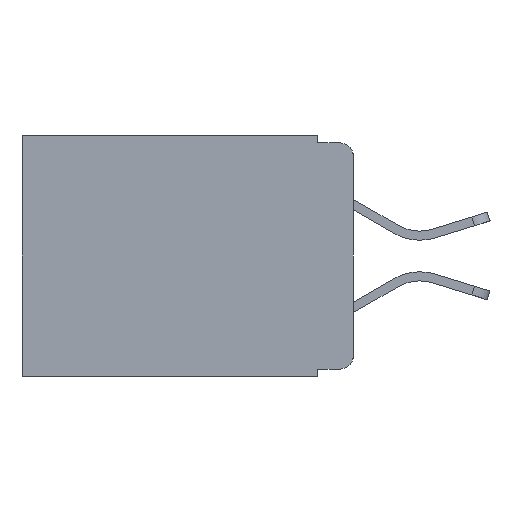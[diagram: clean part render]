
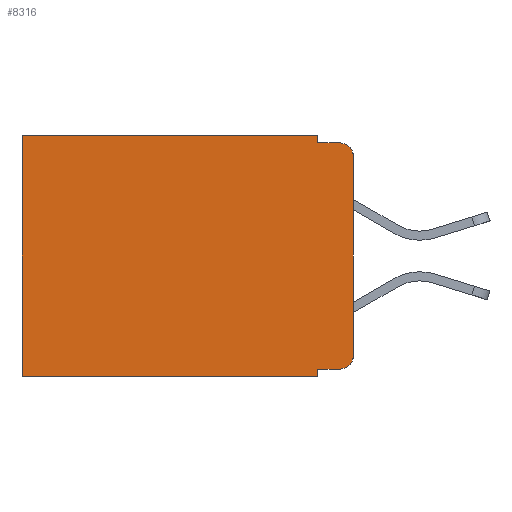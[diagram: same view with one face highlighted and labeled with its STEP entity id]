
A CAD part, left-side view. The second image highlights one B-rep face of the part: STEP entity #8316.
In plain terms, the highlighted planar face has unit normal (-1, 0, 0).
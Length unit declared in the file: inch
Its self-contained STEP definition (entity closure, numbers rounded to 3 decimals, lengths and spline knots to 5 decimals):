
#5 = CARTESIAN_POINT ( 'NONE',  ( 0.298, 0.051, 0. ) ) ;
#56 = ORIENTED_EDGE ( 'NONE', *, *, #6214, .F. ) ;
#148 = CARTESIAN_POINT ( 'NONE',  ( 0.298, 0.051, -0.343 ) ) ;
#188 = ORIENTED_EDGE ( 'NONE', *, *, #1079, .T. ) ;
#370 = VERTEX_POINT ( 'NONE', #11473 ) ;
#743 = CARTESIAN_POINT ( 'NONE',  ( 0.298, 0.02, -0.01 ) ) ;
#910 = ORIENTED_EDGE ( 'NONE', *, *, #11349, .F. ) ;
#989 = CARTESIAN_POINT ( 'NONE',  ( 0.298, 0.473, 0. ) ) ;
#1079 = EDGE_CURVE ( 'NONE', #370, #7854, #6507, .T. ) ;
#1221 = CARTESIAN_POINT ( 'NONE',  ( 0.298, 0., -0.343 ) ) ;
#1286 = VECTOR ( 'NONE', #9434, 39.37008 ) ;
#1333 = VERTEX_POINT ( 'NONE', #9067 ) ;
#2003 = DIRECTION ( 'NONE',  ( 1., 0., 0. ) ) ;
#2022 = ORIENTED_EDGE ( 'NONE', *, *, #6976, .T. ) ;
#2435 = VERTEX_POINT ( 'NONE', #7160 ) ;
#2504 = CARTESIAN_POINT ( 'NONE',  ( 0.298, 0.02, -0.313 ) ) ;
#2575 = VERTEX_POINT ( 'NONE', #5625 ) ;
#2778 = CIRCLE ( 'NONE', #4628, 0.02 ) ;
#2882 = EDGE_CURVE ( 'NONE', #11834, #12901, #2778, .T. ) ;
#3045 = ORIENTED_EDGE ( 'NONE', *, *, #3736, .T. ) ;
#3244 = LINE ( 'NONE', #14928, #9996 ) ;
#3254 = ORIENTED_EDGE ( 'NONE', *, *, #2882, .T. ) ;
#3736 = EDGE_CURVE ( 'NONE', #1333, #11834, #12272, .T. ) ;
#3749 = CARTESIAN_POINT ( 'NONE',  ( 0.298, 0.051, -0.333 ) ) ;
#4028 = VERTEX_POINT ( 'NONE', #8683 ) ;
#4628 = AXIS2_PLACEMENT_3D ( 'NONE', #2504, #8493, #14210 ) ;
#4720 = DIRECTION ( 'NONE',  ( 0., 1., 0. ) ) ;
#4966 = LINE ( 'NONE', #989, #1286 ) ;
#5061 = ORIENTED_EDGE ( 'NONE', *, *, #6609, .F. ) ;
#5110 = LINE ( 'NONE', #1221, #7870 ) ;
#5327 = AXIS2_PLACEMENT_3D ( 'NONE', #6891, #2003, #10416 ) ;
#5462 = ORIENTED_EDGE ( 'NONE', *, *, #7741, .F. ) ;
#5513 = CARTESIAN_POINT ( 'NONE',  ( 0.298, 0., -0.313 ) ) ;
#5625 = CARTESIAN_POINT ( 'NONE',  ( 0.298, 0.473, -0.343 ) ) ;
#6031 = CARTESIAN_POINT ( 'NONE',  ( 0.298, 0., 0. ) ) ;
#6080 = CIRCLE ( 'NONE', #13099, 0.02 ) ;
#6214 = EDGE_CURVE ( 'NONE', #1333, #12821, #9624, .T. ) ;
#6305 = ORIENTED_EDGE ( 'NONE', *, *, #9299, .T. ) ;
#6428 = DIRECTION ( 'NONE',  ( -1., 0., 0. ) ) ;
#6507 = LINE ( 'NONE', #6031, #8857 ) ;
#6540 = VECTOR ( 'NONE', #14878, 39.37008 ) ;
#6609 = EDGE_CURVE ( 'NONE', #4028, #12901, #3244, .T. ) ;
#6891 = CARTESIAN_POINT ( 'NONE',  ( 0.298, 0., 0. ) ) ;
#6976 = EDGE_CURVE ( 'NONE', #7854, #2575, #4966, .T. ) ;
#7160 = CARTESIAN_POINT ( 'NONE',  ( 0.298, 0.051, -0.01 ) ) ;
#7712 = CARTESIAN_POINT ( 'NONE',  ( 0.298, 0.051, 0. ) ) ;
#7741 = EDGE_CURVE ( 'NONE', #370, #2435, #14767, .T. ) ;
#7854 = VERTEX_POINT ( 'NONE', #14893 ) ;
#7870 = VECTOR ( 'NONE', #9661, 39.37008 ) ;
#8039 = PLANE ( 'NONE',  #5327 ) ;
#8294 = VECTOR ( 'NONE', #11265, 39.37008 ) ;
#8316 = ADVANCED_FACE ( 'NONE', ( #14920 ), #8039, .F. ) ;
#8493 = DIRECTION ( 'NONE',  ( -1., 0., 0. ) ) ;
#8542 = EDGE_CURVE ( 'NONE', #2435, #8965, #12496, .T. ) ;
#8683 = CARTESIAN_POINT ( 'NONE',  ( 0.298, 0., -0.03 ) ) ;
#8857 = VECTOR ( 'NONE', #4720, 39.37008 ) ;
#8965 = VERTEX_POINT ( 'NONE', #743 ) ;
#9067 = CARTESIAN_POINT ( 'NONE',  ( 0.298, 0.051, -0.333 ) ) ;
#9299 = EDGE_CURVE ( 'NONE', #4028, #8965, #6080, .T. ) ;
#9434 = DIRECTION ( 'NONE',  ( 0., 0., -1. ) ) ;
#9624 = LINE ( 'NONE', #5, #6540 ) ;
#9661 = DIRECTION ( 'NONE',  ( 0., 1., 0. ) ) ;
#9996 = VECTOR ( 'NONE', #10954, 39.37008 ) ;
#10031 = DIRECTION ( 'NONE',  ( 0., -1., 0. ) ) ;
#10416 = DIRECTION ( 'NONE',  ( 0., 0., -1. ) ) ;
#10954 = DIRECTION ( 'NONE',  ( 0., 0., -1. ) ) ;
#11265 = DIRECTION ( 'NONE',  ( 0., 0., -1. ) ) ;
#11349 = EDGE_CURVE ( 'NONE', #12821, #2575, #5110, .T. ) ;
#11473 = CARTESIAN_POINT ( 'NONE',  ( 0.298, 0.051, 0. ) ) ;
#11767 = CARTESIAN_POINT ( 'NONE',  ( 0.298, 0.02, -0.333 ) ) ;
#11834 = VERTEX_POINT ( 'NONE', #11767 ) ;
#11965 = CARTESIAN_POINT ( 'NONE',  ( 0.298, 0.051, -0.01 ) ) ;
#12272 = LINE ( 'NONE', #3749, #14856 ) ;
#12496 = LINE ( 'NONE', #11965, #15079 ) ;
#12821 = VERTEX_POINT ( 'NONE', #148 ) ;
#12901 = VERTEX_POINT ( 'NONE', #5513 ) ;
#13099 = AXIS2_PLACEMENT_3D ( 'NONE', #13387, #6428, #14488 ) ;
#13252 = EDGE_LOOP ( 'NONE', ( #5061, #6305, #13629, #5462, #188, #2022, #910, #56, #3045, #3254 ) ) ;
#13387 = CARTESIAN_POINT ( 'NONE',  ( 0.298, 0.02, -0.03 ) ) ;
#13629 = ORIENTED_EDGE ( 'NONE', *, *, #8542, .F. ) ;
#14210 = DIRECTION ( 'NONE',  ( 0., 0., -1. ) ) ;
#14226 = DIRECTION ( 'NONE',  ( 0., -1., 0. ) ) ;
#14488 = DIRECTION ( 'NONE',  ( 0., 0., -1. ) ) ;
#14767 = LINE ( 'NONE', #7712, #8294 ) ;
#14856 = VECTOR ( 'NONE', #10031, 39.37008 ) ;
#14878 = DIRECTION ( 'NONE',  ( 0., 0., -1. ) ) ;
#14893 = CARTESIAN_POINT ( 'NONE',  ( 0.298, 0.473, 0. ) ) ;
#14920 = FACE_OUTER_BOUND ( 'NONE', #13252, .T. ) ;
#14928 = CARTESIAN_POINT ( 'NONE',  ( 0.298, 0., 0. ) ) ;
#15079 = VECTOR ( 'NONE', #14226, 39.37008 ) ;
